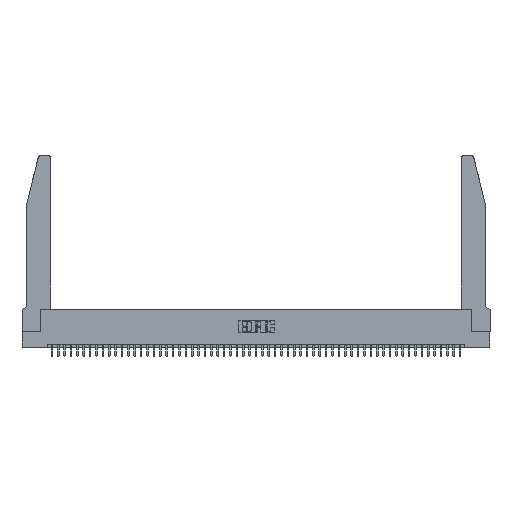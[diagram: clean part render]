
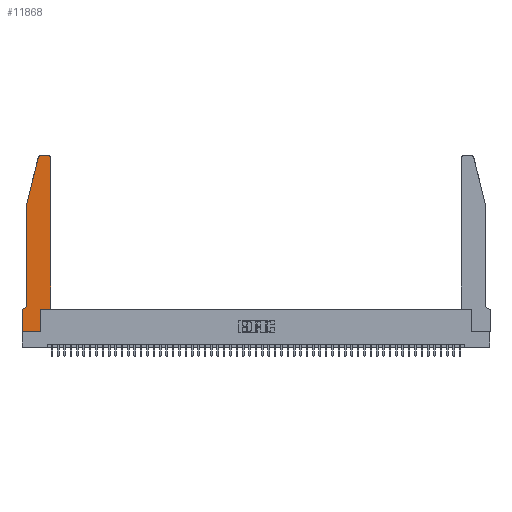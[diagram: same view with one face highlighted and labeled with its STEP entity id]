
A CAD part, top view. The second image highlights one B-rep face of the part: STEP entity #11868.
In plain terms, the highlighted planar face has unit normal (0, 0, 1).
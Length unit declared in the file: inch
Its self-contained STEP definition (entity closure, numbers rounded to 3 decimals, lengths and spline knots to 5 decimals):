
#91 = DIRECTION ( 'NONE',  ( 0., -1., 0. ) ) ;
#534 = CARTESIAN_POINT ( 'NONE',  ( 0.4505, 0.35, 0.37 ) ) ;
#1829 = CARTESIAN_POINT ( 'NONE',  ( 0.0755, 2., 0.37 ) ) ;
#3430 = DIRECTION ( 'NONE',  ( -1., 0., 0. ) ) ;
#3577 = CARTESIAN_POINT ( 'NONE',  ( 0., 0.35, 0.37 ) ) ;
#4115 = ORIENTED_EDGE ( 'NONE', *, *, #45171, .T. ) ;
#4712 = DIRECTION ( 'NONE',  ( 0., 1., 0. ) ) ;
#5060 = VERTEX_POINT ( 'NONE', #21504 ) ;
#5128 = VERTEX_POINT ( 'NONE', #50080 ) ;
#5526 = LINE ( 'NONE', #44671, #47509 ) ;
#5721 = CARTESIAN_POINT ( 'NONE',  ( 0.2865, 0.35, 0.37 ) ) ;
#5940 = ORIENTED_EDGE ( 'NONE', *, *, #16438, .T. ) ;
#6220 = VERTEX_POINT ( 'NONE', #43351 ) ;
#6500 = VERTEX_POINT ( 'NONE', #16663 ) ;
#6528 = DIRECTION ( 'NONE',  ( 0., 0., 1. ) ) ;
#6672 = VERTEX_POINT ( 'NONE', #41885 ) ;
#7033 = VERTEX_POINT ( 'NONE', #11422 ) ;
#7111 = VERTEX_POINT ( 'NONE', #3577 ) ;
#7643 = ORIENTED_EDGE ( 'NONE', *, *, #17415, .T. ) ;
#8642 = VERTEX_POINT ( 'NONE', #47203 ) ;
#9330 = CARTESIAN_POINT ( 'NONE',  ( 0.4205, 2.72, 0.37 ) ) ;
#10048 = CARTESIAN_POINT ( 'NONE',  ( 0.2605, 2.75, 0.37 ) ) ;
#10286 = EDGE_CURVE ( 'NONE', #7111, #6672, #38354, .T. ) ;
#11054 = CIRCLE ( 'NONE', #32436, 0.03 ) ;
#11422 = CARTESIAN_POINT ( 'NONE',  ( 0.0755, 2., 0.37 ) ) ;
#11868 = ADVANCED_FACE ( 'NONE', ( #14154 ), #42038, .T. ) ;
#12066 = EDGE_CURVE ( 'NONE', #6672, #17766, #16050, .T. ) ;
#13510 = DIRECTION ( 'NONE',  ( 1., 0., 0. ) ) ;
#14154 = FACE_OUTER_BOUND ( 'NONE', #41716, .T. ) ;
#16050 = LINE ( 'NONE', #51196, #17313 ) ;
#16438 = EDGE_CURVE ( 'NONE', #6500, #27359, #26171, .T. ) ;
#16663 = CARTESIAN_POINT ( 'NONE',  ( 0.2865, 0.35, 0.37 ) ) ;
#17313 = VECTOR ( 'NONE', #47174, 39.37008 ) ;
#17415 = EDGE_CURVE ( 'NONE', #34295, #7111, #45065, .T. ) ;
#17434 = DIRECTION ( 'NONE',  ( 1., 0., 0. ) ) ;
#17766 = VERTEX_POINT ( 'NONE', #47195 ) ;
#19502 = ORIENTED_EDGE ( 'NONE', *, *, #21846, .T. ) ;
#19800 = LINE ( 'NONE', #5721, #39968 ) ;
#19897 = CARTESIAN_POINT ( 'NONE',  ( 0.0055, 0.35, 0.37 ) ) ;
#20060 = VERTEX_POINT ( 'NONE', #41654 ) ;
#20707 = EDGE_CURVE ( 'NONE', #20060, #5060, #44831, .T. ) ;
#21204 = DIRECTION ( 'NONE',  ( 0., 0., -1. ) ) ;
#21296 = CIRCLE ( 'NONE', #51269, 0.07 ) ;
#21504 = CARTESIAN_POINT ( 'NONE',  ( 0.284, 2.75, 0.37 ) ) ;
#21846 = EDGE_CURVE ( 'NONE', #6220, #34295, #21296, .T. ) ;
#21907 = DIRECTION ( 'NONE',  ( 1., 0., 0. ) ) ;
#22342 = DIRECTION ( 'NONE',  ( -1., 0., 0. ) ) ;
#23263 = CARTESIAN_POINT ( 'NONE',  ( 0.4505, 0.35, 0.37 ) ) ;
#24669 = ORIENTED_EDGE ( 'NONE', *, *, #10286, .T. ) ;
#26171 = LINE ( 'NONE', #37530, #46414 ) ;
#26355 = VECTOR ( 'NONE', #37640, 39.37008 ) ;
#26733 = ORIENTED_EDGE ( 'NONE', *, *, #38376, .T. ) ;
#27359 = VERTEX_POINT ( 'NONE', #23263 ) ;
#27742 = EDGE_CURVE ( 'NONE', #8642, #20060, #43109, .T. ) ;
#28222 = LINE ( 'NONE', #1829, #48475 ) ;
#30893 = CARTESIAN_POINT ( 'NONE',  ( 0.284, 2.72, 0.37 ) ) ;
#31981 = CARTESIAN_POINT ( 'NONE',  ( 0.0755, 0.35, 0.37 ) ) ;
#32436 = AXIS2_PLACEMENT_3D ( 'NONE', #30893, #6528, #34974 ) ;
#32988 = VECTOR ( 'NONE', #3430, 39.37008 ) ;
#33560 = CARTESIAN_POINT ( 'NONE',  ( 0., 0., 0.37 ) ) ;
#34028 = VECTOR ( 'NONE', #22342, 39.37008 ) ;
#34295 = VERTEX_POINT ( 'NONE', #19897 ) ;
#34494 = DIRECTION ( 'NONE',  ( -0.239, -0.971, 0. ) ) ;
#34974 = DIRECTION ( 'NONE',  ( 1., 0., 0. ) ) ;
#35676 = EDGE_CURVE ( 'NONE', #7033, #6220, #5526, .T. ) ;
#37530 = CARTESIAN_POINT ( 'NONE',  ( 0.4505, 0.35, 0.37 ) ) ;
#37640 = DIRECTION ( 'NONE',  ( 0., -1., 0. ) ) ;
#37682 = DIRECTION ( 'NONE',  ( 0., 0., 1. ) ) ;
#38016 = ORIENTED_EDGE ( 'NONE', *, *, #35676, .T. ) ;
#38354 = LINE ( 'NONE', #33560, #26355 ) ;
#38376 = EDGE_CURVE ( 'NONE', #5128, #7033, #28222, .T. ) ;
#38389 = ORIENTED_EDGE ( 'NONE', *, *, #51895, .T. ) ;
#39968 = VECTOR ( 'NONE', #50269, 39.37008 ) ;
#40823 = AXIS2_PLACEMENT_3D ( 'NONE', #45944, #46107, #21907 ) ;
#41146 = ORIENTED_EDGE ( 'NONE', *, *, #20707, .T. ) ;
#41654 = CARTESIAN_POINT ( 'NONE',  ( 0.4205, 2.75, 0.37 ) ) ;
#41716 = EDGE_LOOP ( 'NONE', ( #41146, #42591, #26733, #38016, #19502, #7643, #24669, #45911, #4115, #5940, #38389, #43909 ) ) ;
#41885 = CARTESIAN_POINT ( 'NONE',  ( 0., 0., 0.37 ) ) ;
#42038 = PLANE ( 'NONE',  #40823 ) ;
#42591 = ORIENTED_EDGE ( 'NONE', *, *, #49150, .T. ) ;
#43109 = CIRCLE ( 'NONE', #47744, 0.03 ) ;
#43351 = CARTESIAN_POINT ( 'NONE',  ( 0.0755, 0.42, 0.37 ) ) ;
#43909 = ORIENTED_EDGE ( 'NONE', *, *, #27742, .T. ) ;
#44671 = CARTESIAN_POINT ( 'NONE',  ( 0.0755, 2., 0.37 ) ) ;
#44698 = VECTOR ( 'NONE', #4712, 39.37008 ) ;
#44831 = LINE ( 'NONE', #10048, #34028 ) ;
#45065 = LINE ( 'NONE', #31981, #32988 ) ;
#45171 = EDGE_CURVE ( 'NONE', #17766, #6500, #19800, .T. ) ;
#45403 = CARTESIAN_POINT ( 'NONE',  ( 0.0055, 0.42, 0.37 ) ) ;
#45911 = ORIENTED_EDGE ( 'NONE', *, *, #12066, .T. ) ;
#45944 = CARTESIAN_POINT ( 'NONE',  ( 0., 0.35, 0.37 ) ) ;
#45948 = LINE ( 'NONE', #534, #44698 ) ;
#46107 = DIRECTION ( 'NONE',  ( 0., 0., 1. ) ) ;
#46414 = VECTOR ( 'NONE', #17434, 39.37008 ) ;
#47174 = DIRECTION ( 'NONE',  ( 1., 0., 0. ) ) ;
#47195 = CARTESIAN_POINT ( 'NONE',  ( 0.2865, 0., 0.37 ) ) ;
#47203 = CARTESIAN_POINT ( 'NONE',  ( 0.4505, 2.72, 0.37 ) ) ;
#47509 = VECTOR ( 'NONE', #91, 39.37008 ) ;
#47744 = AXIS2_PLACEMENT_3D ( 'NONE', #9330, #37682, #13510 ) ;
#48475 = VECTOR ( 'NONE', #34494, 39.37008 ) ;
#49150 = EDGE_CURVE ( 'NONE', #5060, #5128, #11054, .T. ) ;
#49422 = DIRECTION ( 'NONE',  ( -1., 0., 0. ) ) ;
#50080 = CARTESIAN_POINT ( 'NONE',  ( 0.25487, 2.72718, 0.37 ) ) ;
#50269 = DIRECTION ( 'NONE',  ( 0., 1., 0. ) ) ;
#51196 = CARTESIAN_POINT ( 'NONE',  ( 0., 0., 0.37 ) ) ;
#51269 = AXIS2_PLACEMENT_3D ( 'NONE', #45403, #21204, #49422 ) ;
#51895 = EDGE_CURVE ( 'NONE', #27359, #8642, #45948, .T. ) ;
